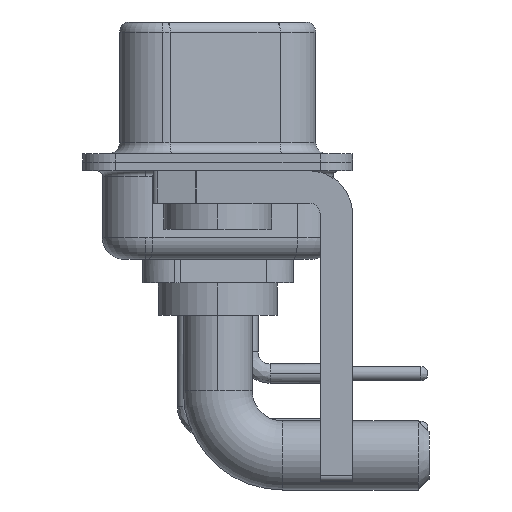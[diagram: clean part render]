
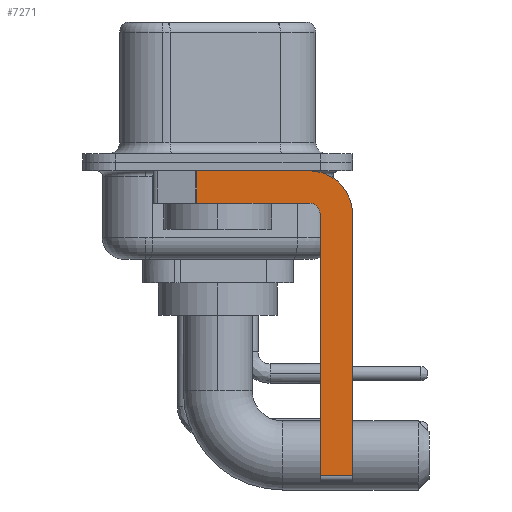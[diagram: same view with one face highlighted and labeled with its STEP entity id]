
A CAD part, left-side view. The second image highlights one B-rep face of the part: STEP entity #7271.
In plain terms, the highlighted planar face has unit normal (-1, 0, 0).
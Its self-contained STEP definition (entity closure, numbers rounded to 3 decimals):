
#760 = ORIENTED_EDGE ( 'NONE', *, *, #15165, .F. ) ;
#806 = CIRCLE ( 'NONE', #19854, 2. ) ;
#827 = VERTEX_POINT ( 'NONE', #16614 ) ;
#876 = VECTOR ( 'NONE', #15372, 1000. ) ;
#1438 = CARTESIAN_POINT ( 'NONE',  ( -2.9, 0.978, -0.4 ) ) ;
#1587 = CARTESIAN_POINT ( 'NONE',  ( -2.9, -4.25, -2.4 ) ) ;
#1700 = DIRECTION ( 'NONE',  ( 0., 0., 1. ) ) ;
#1818 = CIRCLE ( 'NONE', #2321, 0.5 ) ;
#2188 = FACE_OUTER_BOUND ( 'NONE', #6526, .T. ) ;
#2321 = AXIS2_PLACEMENT_3D ( 'NONE', #8023, #15025, #19228 ) ;
#2576 = CARTESIAN_POINT ( 'NONE',  ( -2.9, -6.25, -2.4 ) ) ;
#3088 = CARTESIAN_POINT ( 'NONE',  ( -2.9, 0.978, -1.9 ) ) ;
#3688 = VERTEX_POINT ( 'NONE', #8425 ) ;
#4027 = LINE ( 'NONE', #17307, #26813 ) ;
#4110 = DIRECTION ( 'NONE',  ( 0., 0., -1. ) ) ;
#4575 = LINE ( 'NONE', #11245, #9035 ) ;
#4676 = DIRECTION ( 'NONE',  ( 1., 0., 0. ) ) ;
#5991 = CARTESIAN_POINT ( 'NONE',  ( -2.9, -6.25, -2.4 ) ) ;
#6526 = EDGE_LOOP ( 'NONE', ( #20330, #22630, #760, #13978, #9548, #24987, #21955, #23902 ) ) ;
#6856 = CARTESIAN_POINT ( 'NONE',  ( -2.9, -4.25, -1.9 ) ) ;
#7271 = ADVANCED_FACE ( 'NONE', ( #2188 ), #29322, .F. ) ;
#7740 = EDGE_CURVE ( 'NONE', #3688, #9299, #24348, .T. ) ;
#8023 = CARTESIAN_POINT ( 'NONE',  ( -2.9, -4.25, -2.4 ) ) ;
#8425 = CARTESIAN_POINT ( 'NONE',  ( -2.9, -4.75, -14.55 ) ) ;
#8721 = DIRECTION ( 'NONE',  ( 0., -1., 0. ) ) ;
#8950 = CARTESIAN_POINT ( 'NONE',  ( -2.9, 0.978, -1.9 ) ) ;
#9035 = VECTOR ( 'NONE', #8721, 1000. ) ;
#9299 = VERTEX_POINT ( 'NONE', #9968 ) ;
#9548 = ORIENTED_EDGE ( 'NONE', *, *, #7740, .F. ) ;
#9550 = DIRECTION ( 'NONE',  ( 0., 0., -1. ) ) ;
#9640 = DIRECTION ( 'NONE',  ( 0., 0., -1. ) ) ;
#9968 = CARTESIAN_POINT ( 'NONE',  ( -2.9, -4.75, -2.4 ) ) ;
#11245 = CARTESIAN_POINT ( 'NONE',  ( -2.9, -4.25, -14.55 ) ) ;
#11849 = EDGE_CURVE ( 'NONE', #19054, #23125, #4027, .T. ) ;
#11938 = VECTOR ( 'NONE', #1700, 1000. ) ;
#13835 = VECTOR ( 'NONE', #9640, 1000. ) ;
#13978 = ORIENTED_EDGE ( 'NONE', *, *, #25261, .F. ) ;
#14663 = EDGE_CURVE ( 'NONE', #14996, #827, #26425, .T. ) ;
#14996 = VERTEX_POINT ( 'NONE', #2576 ) ;
#15025 = DIRECTION ( 'NONE',  ( -1., 0., 0. ) ) ;
#15165 = EDGE_CURVE ( 'NONE', #21034, #18129, #18055, .T. ) ;
#15372 = DIRECTION ( 'NONE',  ( 0., 0., -1. ) ) ;
#15604 = EDGE_CURVE ( 'NONE', #3688, #827, #4575, .T. ) ;
#15641 = DIRECTION ( 'NONE',  ( 0., 1., 0. ) ) ;
#16362 = LINE ( 'NONE', #3088, #13835 ) ;
#16614 = CARTESIAN_POINT ( 'NONE',  ( -2.9, -6.25, -14.55 ) ) ;
#16641 = EDGE_CURVE ( 'NONE', #19054, #18129, #16362, .T. ) ;
#17307 = CARTESIAN_POINT ( 'NONE',  ( -2.9, 3., -0.4 ) ) ;
#18055 = LINE ( 'NONE', #6856, #25201 ) ;
#18129 = VERTEX_POINT ( 'NONE', #8950 ) ;
#19054 = VERTEX_POINT ( 'NONE', #1438 ) ;
#19228 = DIRECTION ( 'NONE',  ( 0., 0., 1. ) ) ;
#19854 = AXIS2_PLACEMENT_3D ( 'NONE', #29424, #4676, #9550 ) ;
#19911 = DIRECTION ( 'NONE',  ( 1., 0., 0. ) ) ;
#20330 = ORIENTED_EDGE ( 'NONE', *, *, #11849, .F. ) ;
#21034 = VERTEX_POINT ( 'NONE', #24847 ) ;
#21955 = ORIENTED_EDGE ( 'NONE', *, *, #14663, .F. ) ;
#22112 = CARTESIAN_POINT ( 'NONE',  ( -2.9, -4.75, -14.8 ) ) ;
#22630 = ORIENTED_EDGE ( 'NONE', *, *, #16641, .T. ) ;
#23125 = VERTEX_POINT ( 'NONE', #29457 ) ;
#23827 = AXIS2_PLACEMENT_3D ( 'NONE', #1587, #19911, #4110 ) ;
#23900 = EDGE_CURVE ( 'NONE', #23125, #14996, #806, .T. ) ;
#23902 = ORIENTED_EDGE ( 'NONE', *, *, #23900, .F. ) ;
#24302 = DIRECTION ( 'NONE',  ( 0., -1., 0. ) ) ;
#24348 = LINE ( 'NONE', #22112, #11938 ) ;
#24847 = CARTESIAN_POINT ( 'NONE',  ( -2.9, -4.25, -1.9 ) ) ;
#24987 = ORIENTED_EDGE ( 'NONE', *, *, #15604, .T. ) ;
#25201 = VECTOR ( 'NONE', #15641, 1000. ) ;
#25261 = EDGE_CURVE ( 'NONE', #9299, #21034, #1818, .T. ) ;
#26425 = LINE ( 'NONE', #5991, #876 ) ;
#26813 = VECTOR ( 'NONE', #24302, 1000. ) ;
#29322 = PLANE ( 'NONE',  #23827 ) ;
#29424 = CARTESIAN_POINT ( 'NONE',  ( -2.9, -4.25, -2.4 ) ) ;
#29457 = CARTESIAN_POINT ( 'NONE',  ( -2.9, -4.25, -0.4 ) ) ;
